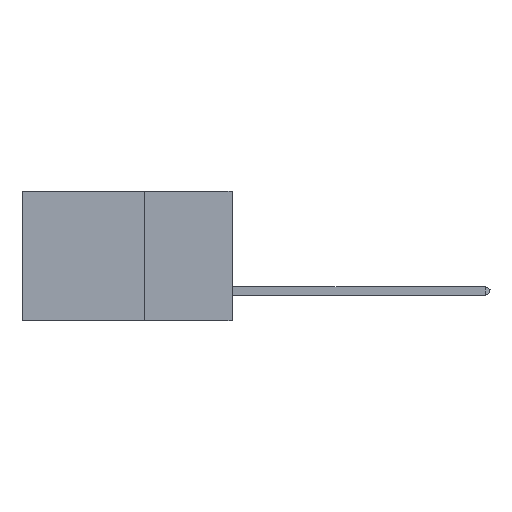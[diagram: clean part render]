
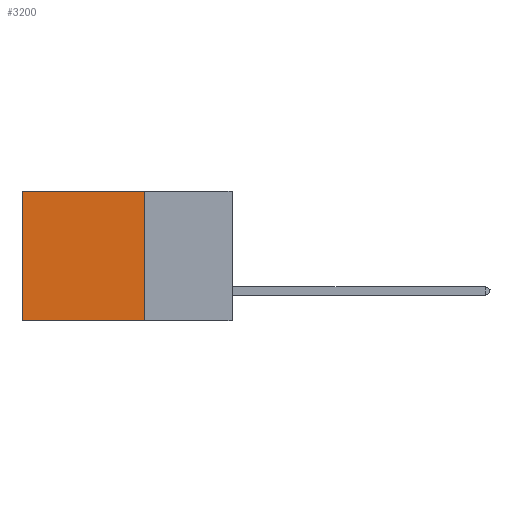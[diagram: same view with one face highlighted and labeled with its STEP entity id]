
A CAD part, left-side view. The second image highlights one B-rep face of the part: STEP entity #3200.
In plain terms, the highlighted planar face has unit normal (-1, 0, 0).
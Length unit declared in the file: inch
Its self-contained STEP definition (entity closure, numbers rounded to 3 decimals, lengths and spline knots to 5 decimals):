
#1173 = VECTOR ( 'NONE', #2114, 39.37008 ) ;
#2033 = CARTESIAN_POINT ( 'NONE',  ( 0.2875, 0.25, 0. ) ) ;
#2114 = DIRECTION ( 'NONE',  ( 0., 1., 0. ) ) ;
#3200 = ADVANCED_FACE ( 'NONE', ( #16064 ), #4942, .F. ) ;
#3632 = DIRECTION ( 'NONE',  ( 0., 1., 0. ) ) ;
#4627 = CARTESIAN_POINT ( 'NONE',  ( 0.2875, 0.25, -0.37 ) ) ;
#4687 = AXIS2_PLACEMENT_3D ( 'NONE', #17160, #5058, #11600 ) ;
#4942 = PLANE ( 'NONE',  #4687 ) ;
#5058 = DIRECTION ( 'NONE',  ( 1., 0., 0. ) ) ;
#5862 = EDGE_CURVE ( 'NONE', #6283, #11931, #6617, .T. ) ;
#6032 = CARTESIAN_POINT ( 'NONE',  ( 0.2875, 0.25, 0. ) ) ;
#6103 = ORIENTED_EDGE ( 'NONE', *, *, #11570, .F. ) ;
#6283 = VERTEX_POINT ( 'NONE', #13411 ) ;
#6351 = LINE ( 'NONE', #6032, #1173 ) ;
#6499 = VECTOR ( 'NONE', #3632, 39.37008 ) ;
#6617 = LINE ( 'NONE', #9714, #9350 ) ;
#7845 = EDGE_LOOP ( 'NONE', ( #11591, #6103, #8505, #14063 ) ) ;
#8505 = ORIENTED_EDGE ( 'NONE', *, *, #16881, .F. ) ;
#8511 = VERTEX_POINT ( 'NONE', #2033 ) ;
#8806 = EDGE_CURVE ( 'NONE', #8511, #6283, #6351, .T. ) ;
#8821 = LINE ( 'NONE', #13500, #6499 ) ;
#9011 = VECTOR ( 'NONE', #13650, 39.37008 ) ;
#9350 = VECTOR ( 'NONE', #14977, 39.37008 ) ;
#9714 = CARTESIAN_POINT ( 'NONE',  ( 0.2875, 0.6, 0. ) ) ;
#11090 = CARTESIAN_POINT ( 'NONE',  ( 0.2875, 0.25, 0. ) ) ;
#11570 = EDGE_CURVE ( 'NONE', #17135, #11931, #8821, .T. ) ;
#11591 = ORIENTED_EDGE ( 'NONE', *, *, #5862, .T. ) ;
#11600 = DIRECTION ( 'NONE',  ( 0., 0., -1. ) ) ;
#11931 = VERTEX_POINT ( 'NONE', #13772 ) ;
#12758 = LINE ( 'NONE', #11090, #9011 ) ;
#13411 = CARTESIAN_POINT ( 'NONE',  ( 0.2875, 0.6, 0. ) ) ;
#13500 = CARTESIAN_POINT ( 'NONE',  ( 0.2875, 0.25, -0.37 ) ) ;
#13650 = DIRECTION ( 'NONE',  ( 0., 0., -1. ) ) ;
#13772 = CARTESIAN_POINT ( 'NONE',  ( 0.2875, 0.6, -0.37 ) ) ;
#14063 = ORIENTED_EDGE ( 'NONE', *, *, #8806, .T. ) ;
#14977 = DIRECTION ( 'NONE',  ( 0., 0., -1. ) ) ;
#16064 = FACE_OUTER_BOUND ( 'NONE', #7845, .T. ) ;
#16881 = EDGE_CURVE ( 'NONE', #8511, #17135, #12758, .T. ) ;
#17135 = VERTEX_POINT ( 'NONE', #4627 ) ;
#17160 = CARTESIAN_POINT ( 'NONE',  ( 0.2875, 0.25, 0. ) ) ;
